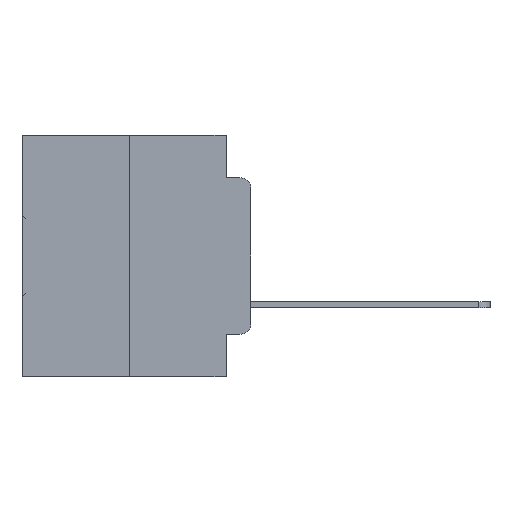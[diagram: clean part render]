
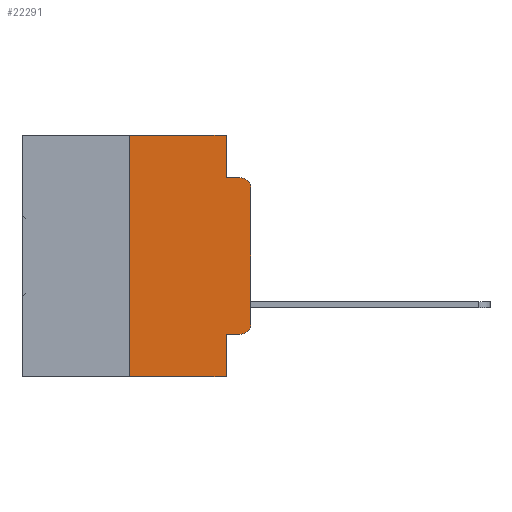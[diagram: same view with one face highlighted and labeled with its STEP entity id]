
A CAD part, left-side view. The second image highlights one B-rep face of the part: STEP entity #22291.
In plain terms, the highlighted planar face has unit normal (-1, 0, 0).
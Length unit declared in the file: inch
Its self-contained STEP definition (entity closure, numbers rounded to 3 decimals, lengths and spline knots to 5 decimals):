
#1576 = DIRECTION ( 'NONE',  ( 0., 0., -1. ) ) ;
#1911 = VECTOR ( 'NONE', #1576, 39.37008 ) ;
#2058 = CARTESIAN_POINT ( 'NONE',  ( 0., 0.051, -0.4115 ) ) ;
#2122 = LINE ( 'NONE', #25742, #10464 ) ;
#2532 = ORIENTED_EDGE ( 'NONE', *, *, #9114, .T. ) ;
#2611 = ORIENTED_EDGE ( 'NONE', *, *, #28505, .F. ) ;
#2717 = VERTEX_POINT ( 'NONE', #15627 ) ;
#3531 = DIRECTION ( 'NONE',  ( 1., 0., 0. ) ) ;
#4088 = CARTESIAN_POINT ( 'NONE',  ( 0., 0.02, -0.4115 ) ) ;
#4415 = LINE ( 'NONE', #2058, #17970 ) ;
#4535 = VERTEX_POINT ( 'NONE', #27070 ) ;
#4754 = CARTESIAN_POINT ( 'NONE',  ( 0., 0.473, 0. ) ) ;
#4917 = DIRECTION ( 'NONE',  ( 0., -1., 0. ) ) ;
#4943 = DIRECTION ( 'NONE',  ( -1., 0., 0. ) ) ;
#5342 = VERTEX_POINT ( 'NONE', #13715 ) ;
#5367 = CARTESIAN_POINT ( 'NONE',  ( 0., 0., -0.1085 ) ) ;
#5615 = LINE ( 'NONE', #15745, #26323 ) ;
#6714 = CARTESIAN_POINT ( 'NONE',  ( 0., 0.051, -0.5 ) ) ;
#7312 = CARTESIAN_POINT ( 'NONE',  ( 0., 0.02, -0.1085 ) ) ;
#7457 = AXIS2_PLACEMENT_3D ( 'NONE', #7312, #25395, #10114 ) ;
#8009 = CARTESIAN_POINT ( 'NONE',  ( 0., 0.051, 0. ) ) ;
#8214 = VERTEX_POINT ( 'NONE', #23198 ) ;
#9114 = EDGE_CURVE ( 'NONE', #2717, #19873, #23648, .T. ) ;
#9819 = DIRECTION ( 'NONE',  ( 0., 0., 1. ) ) ;
#9926 = EDGE_LOOP ( 'NONE', ( #2532, #16741, #13869, #2611, #12621, #28277, #19141, #16799, #13930, #28717 ) ) ;
#10114 = DIRECTION ( 'NONE',  ( 0., 0., -1. ) ) ;
#10464 = VECTOR ( 'NONE', #4917, 39.37008 ) ;
#12621 = ORIENTED_EDGE ( 'NONE', *, *, #33382, .F. ) ;
#13487 = EDGE_CURVE ( 'NONE', #32460, #2717, #13579, .T. ) ;
#13579 = CIRCLE ( 'NONE', #23133, 0.02 ) ;
#13715 = CARTESIAN_POINT ( 'NONE',  ( 0., 0.051, -0.0885 ) ) ;
#13741 = VERTEX_POINT ( 'NONE', #24408 ) ;
#13869 = ORIENTED_EDGE ( 'NONE', *, *, #31730, .F. ) ;
#13930 = ORIENTED_EDGE ( 'NONE', *, *, #15226, .T. ) ;
#14012 = VECTOR ( 'NONE', #25602, 39.37008 ) ;
#15226 = EDGE_CURVE ( 'NONE', #31192, #32460, #4415, .T. ) ;
#15627 = CARTESIAN_POINT ( 'NONE',  ( 0., 0., -0.3915 ) ) ;
#15643 = CIRCLE ( 'NONE', #7457, 0.02 ) ;
#15745 = CARTESIAN_POINT ( 'NONE',  ( 0., 0.25, 0. ) ) ;
#15884 = CARTESIAN_POINT ( 'NONE',  ( 0., 0.051, -0.0885 ) ) ;
#16741 = ORIENTED_EDGE ( 'NONE', *, *, #33320, .T. ) ;
#16799 = ORIENTED_EDGE ( 'NONE', *, *, #16998, .F. ) ;
#16998 = EDGE_CURVE ( 'NONE', #31192, #19470, #25030, .T. ) ;
#17970 = VECTOR ( 'NONE', #18354, 39.37008 ) ;
#18180 = VERTEX_POINT ( 'NONE', #27874 ) ;
#18354 = DIRECTION ( 'NONE',  ( 0., -1., 0. ) ) ;
#19141 = ORIENTED_EDGE ( 'NONE', *, *, #23420, .T. ) ;
#19470 = VERTEX_POINT ( 'NONE', #6714 ) ;
#19634 = CARTESIAN_POINT ( 'NONE',  ( 0., 0.473, 0. ) ) ;
#19873 = VERTEX_POINT ( 'NONE', #5367 ) ;
#20878 = CARTESIAN_POINT ( 'NONE',  ( 0., 0.02, -0.3915 ) ) ;
#21669 = LINE ( 'NONE', #15884, #28890 ) ;
#22032 = FACE_OUTER_BOUND ( 'NONE', #9926, .T. ) ;
#22122 = DIRECTION ( 'NONE',  ( 0., 0., -1. ) ) ;
#22291 = ADVANCED_FACE ( 'NONE', ( #22032 ), #31746, .F. ) ;
#23133 = AXIS2_PLACEMENT_3D ( 'NONE', #20878, #4943, #23340 ) ;
#23198 = CARTESIAN_POINT ( 'NONE',  ( 0., 0.02, -0.0885 ) ) ;
#23340 = DIRECTION ( 'NONE',  ( 0., 0., -1. ) ) ;
#23420 = EDGE_CURVE ( 'NONE', #18180, #19470, #2122, .T. ) ;
#23648 = LINE ( 'NONE', #25141, #30846 ) ;
#23661 = CARTESIAN_POINT ( 'NONE',  ( 0., 0.051, -0.4115 ) ) ;
#24291 = VECTOR ( 'NONE', #26003, 39.37008 ) ;
#24408 = CARTESIAN_POINT ( 'NONE',  ( 0., 0.25, 0. ) ) ;
#25030 = LINE ( 'NONE', #8009, #24291 ) ;
#25141 = CARTESIAN_POINT ( 'NONE',  ( 0., 0., 0. ) ) ;
#25228 = EDGE_CURVE ( 'NONE', #18180, #13741, #5615, .T. ) ;
#25395 = DIRECTION ( 'NONE',  ( -1., 0., 0. ) ) ;
#25602 = DIRECTION ( 'NONE',  ( 0., -1., 0. ) ) ;
#25742 = CARTESIAN_POINT ( 'NONE',  ( 0., 0.473, -0.5 ) ) ;
#26003 = DIRECTION ( 'NONE',  ( 0., 0., -1. ) ) ;
#26323 = VECTOR ( 'NONE', #32867, 39.37008 ) ;
#26765 = AXIS2_PLACEMENT_3D ( 'NONE', #19634, #3531, #22122 ) ;
#27070 = CARTESIAN_POINT ( 'NONE',  ( 0., 0.051, 0. ) ) ;
#27874 = CARTESIAN_POINT ( 'NONE',  ( 0., 0.25, -0.5 ) ) ;
#28277 = ORIENTED_EDGE ( 'NONE', *, *, #25228, .F. ) ;
#28505 = EDGE_CURVE ( 'NONE', #4535, #5342, #29591, .T. ) ;
#28717 = ORIENTED_EDGE ( 'NONE', *, *, #13487, .T. ) ;
#28890 = VECTOR ( 'NONE', #30604, 39.37008 ) ;
#29535 = LINE ( 'NONE', #4754, #14012 ) ;
#29591 = LINE ( 'NONE', #32522, #1911 ) ;
#30604 = DIRECTION ( 'NONE',  ( 0., -1., 0. ) ) ;
#30846 = VECTOR ( 'NONE', #9819, 39.37008 ) ;
#31192 = VERTEX_POINT ( 'NONE', #23661 ) ;
#31730 = EDGE_CURVE ( 'NONE', #5342, #8214, #21669, .T. ) ;
#31746 = PLANE ( 'NONE',  #26765 ) ;
#32460 = VERTEX_POINT ( 'NONE', #4088 ) ;
#32522 = CARTESIAN_POINT ( 'NONE',  ( 0., 0.051, 0. ) ) ;
#32867 = DIRECTION ( 'NONE',  ( 0., 0., 1. ) ) ;
#33320 = EDGE_CURVE ( 'NONE', #19873, #8214, #15643, .T. ) ;
#33382 = EDGE_CURVE ( 'NONE', #13741, #4535, #29535, .T. ) ;
